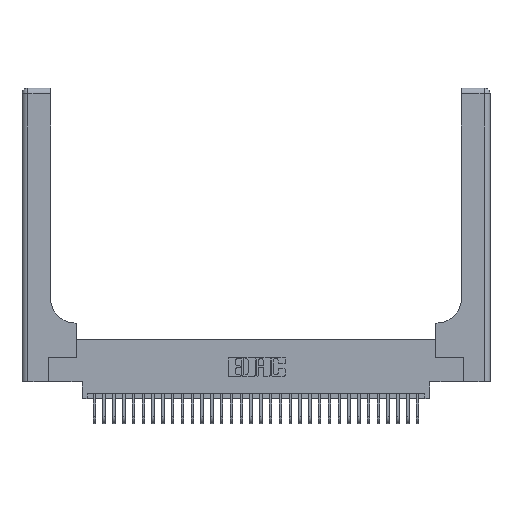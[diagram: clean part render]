
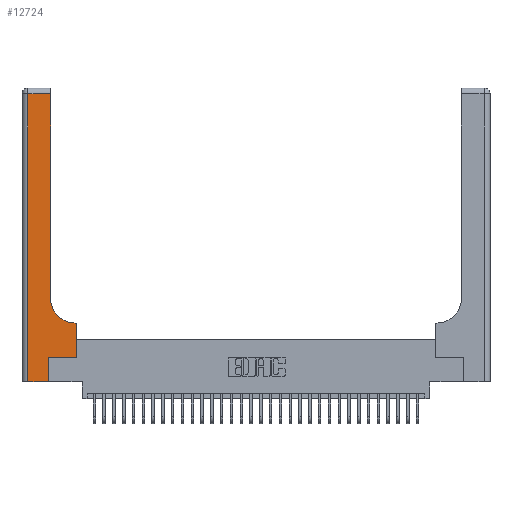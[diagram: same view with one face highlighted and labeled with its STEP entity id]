
A CAD part, top view. The second image highlights one B-rep face of the part: STEP entity #12724.
In plain terms, the highlighted planar face has unit normal (0, 0, 1).
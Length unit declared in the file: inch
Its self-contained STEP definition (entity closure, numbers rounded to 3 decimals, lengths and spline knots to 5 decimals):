
#738 = VECTOR ( 'NONE', #1759, 39.37008 ) ;
#771 = DIRECTION ( 'NONE',  ( 1., 0., 0. ) ) ;
#1142 = CARTESIAN_POINT ( 'NONE',  ( 0.5415, 0.85, 0.37 ) ) ;
#1478 = EDGE_CURVE ( 'NONE', #18863, #13312, #24311, .T. ) ;
#1622 = CARTESIAN_POINT ( 'NONE',  ( 0.269, 0.25, 0.37 ) ) ;
#1723 = VERTEX_POINT ( 'NONE', #4555 ) ;
#1759 = DIRECTION ( 'NONE',  ( 0., -1., 0. ) ) ;
#2734 = CARTESIAN_POINT ( 'NONE',  ( 0., 2.94, 0.37 ) ) ;
#2943 = DIRECTION ( 'NONE',  ( 0., 1., 0. ) ) ;
#3087 = VECTOR ( 'NONE', #8475, 39.37008 ) ;
#3121 = VERTEX_POINT ( 'NONE', #8163 ) ;
#3489 = CARTESIAN_POINT ( 'NONE',  ( 0.269, 0.25, 0.37 ) ) ;
#3706 = DIRECTION ( 'NONE',  ( 1., 0., 0. ) ) ;
#4280 = PLANE ( 'NONE',  #7891 ) ;
#4555 = CARTESIAN_POINT ( 'NONE',  ( 0.2915, 0.85, 0.37 ) ) ;
#5199 = VECTOR ( 'NONE', #2943, 39.37008 ) ;
#5327 = ORIENTED_EDGE ( 'NONE', *, *, #31291, .T. ) ;
#6118 = FACE_OUTER_BOUND ( 'NONE', #19067, .T. ) ;
#6641 = CARTESIAN_POINT ( 'NONE',  ( 0.06, 0., 0.37 ) ) ;
#6778 = DIRECTION ( 'NONE',  ( -1., 0., 0. ) ) ;
#6955 = CARTESIAN_POINT ( 'NONE',  ( 0.5585, 0.25, 0.37 ) ) ;
#7254 = VECTOR ( 'NONE', #771, 39.37008 ) ;
#7891 = AXIS2_PLACEMENT_3D ( 'NONE', #31328, #21524, #6778 ) ;
#8163 = CARTESIAN_POINT ( 'NONE',  ( 0.06, 2.94, 0.37 ) ) ;
#8475 = DIRECTION ( 'NONE',  ( 1., 0., 0. ) ) ;
#9590 = EDGE_CURVE ( 'NONE', #13312, #17737, #11809, .T. ) ;
#10201 = VECTOR ( 'NONE', #29183, 39.37008 ) ;
#10514 = CARTESIAN_POINT ( 'NONE',  ( 0.269, 0., 0.37 ) ) ;
#10515 = VECTOR ( 'NONE', #28796, 39.37008 ) ;
#10536 = EDGE_CURVE ( 'NONE', #19768, #18863, #30586, .T. ) ;
#11087 = VERTEX_POINT ( 'NONE', #28490 ) ;
#11115 = ORIENTED_EDGE ( 'NONE', *, *, #30633, .T. ) ;
#11275 = LINE ( 'NONE', #31271, #10515 ) ;
#11623 = EDGE_CURVE ( 'NONE', #1723, #23048, #11275, .T. ) ;
#11809 = LINE ( 'NONE', #27644, #5199 ) ;
#12724 = ADVANCED_FACE ( 'NONE', ( #6118 ), #4280, .F. ) ;
#13312 = VERTEX_POINT ( 'NONE', #6955 ) ;
#13841 = LINE ( 'NONE', #2734, #26894 ) ;
#14022 = LINE ( 'NONE', #31343, #738 ) ;
#14339 = ORIENTED_EDGE ( 'NONE', *, *, #26285, .T. ) ;
#15359 = ORIENTED_EDGE ( 'NONE', *, *, #9590, .T. ) ;
#16029 = CARTESIAN_POINT ( 'NONE',  ( 0.2915, 0.6, 0.37 ) ) ;
#16146 = DIRECTION ( 'NONE',  ( -1., 0., 0. ) ) ;
#17737 = VERTEX_POINT ( 'NONE', #25737 ) ;
#18087 = ORIENTED_EDGE ( 'NONE', *, *, #22363, .T. ) ;
#18463 = ORIENTED_EDGE ( 'NONE', *, *, #21106, .T. ) ;
#18529 = DIRECTION ( 'NONE',  ( 0., 0., -1. ) ) ;
#18863 = VERTEX_POINT ( 'NONE', #1622 ) ;
#19067 = EDGE_LOOP ( 'NONE', ( #30344, #11115, #18087, #5327, #25437, #19755, #15359, #18463, #14339 ) ) ;
#19755 = ORIENTED_EDGE ( 'NONE', *, *, #1478, .T. ) ;
#19768 = VERTEX_POINT ( 'NONE', #10514 ) ;
#19914 = CIRCLE ( 'NONE', #21776, 0.25 ) ;
#19955 = LINE ( 'NONE', #30421, #7254 ) ;
#21106 = EDGE_CURVE ( 'NONE', #17737, #11087, #30954, .T. ) ;
#21524 = DIRECTION ( 'NONE',  ( 0., 0., -1. ) ) ;
#21776 = AXIS2_PLACEMENT_3D ( 'NONE', #1142, #18529, #3706 ) ;
#22363 = EDGE_CURVE ( 'NONE', #3121, #24583, #14022, .T. ) ;
#23048 = VERTEX_POINT ( 'NONE', #24084 ) ;
#24084 = CARTESIAN_POINT ( 'NONE',  ( 0.2915, 2.94, 0.37 ) ) ;
#24311 = LINE ( 'NONE', #3489, #3087 ) ;
#24583 = VERTEX_POINT ( 'NONE', #6641 ) ;
#25437 = ORIENTED_EDGE ( 'NONE', *, *, #10536, .T. ) ;
#25737 = CARTESIAN_POINT ( 'NONE',  ( 0.5585, 0.6, 0.37 ) ) ;
#26285 = EDGE_CURVE ( 'NONE', #11087, #1723, #19914, .T. ) ;
#26697 = CARTESIAN_POINT ( 'NONE',  ( 0.269, 0., 0.37 ) ) ;
#26894 = VECTOR ( 'NONE', #29908, 39.37008 ) ;
#27644 = CARTESIAN_POINT ( 'NONE',  ( 0.5585, 0.25, 0.37 ) ) ;
#28490 = CARTESIAN_POINT ( 'NONE',  ( 0.5415, 0.6, 0.37 ) ) ;
#28796 = DIRECTION ( 'NONE',  ( 0., 1., 0. ) ) ;
#29183 = DIRECTION ( 'NONE',  ( 0., 1., 0. ) ) ;
#29908 = DIRECTION ( 'NONE',  ( -1., 0., 0. ) ) ;
#30199 = VECTOR ( 'NONE', #16146, 39.37008 ) ;
#30344 = ORIENTED_EDGE ( 'NONE', *, *, #11623, .T. ) ;
#30421 = CARTESIAN_POINT ( 'NONE',  ( 0., 0., 0.37 ) ) ;
#30586 = LINE ( 'NONE', #26697, #10201 ) ;
#30633 = EDGE_CURVE ( 'NONE', #23048, #3121, #13841, .T. ) ;
#30954 = LINE ( 'NONE', #16029, #30199 ) ;
#31271 = CARTESIAN_POINT ( 'NONE',  ( 0.2915, 3., 0.37 ) ) ;
#31291 = EDGE_CURVE ( 'NONE', #24583, #19768, #19955, .T. ) ;
#31328 = CARTESIAN_POINT ( 'NONE',  ( 0., 3., 0.37 ) ) ;
#31343 = CARTESIAN_POINT ( 'NONE',  ( 0.06, 3., 0.37 ) ) ;
